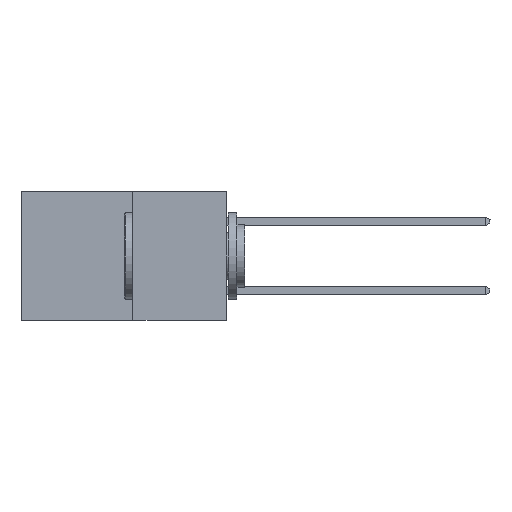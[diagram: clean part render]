
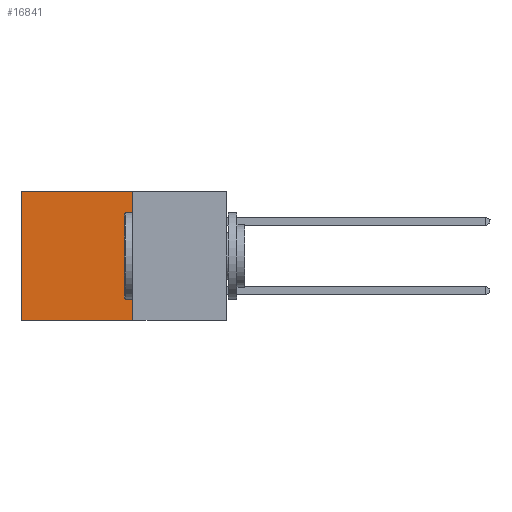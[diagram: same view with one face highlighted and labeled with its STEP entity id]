
A CAD part, left-side view. The second image highlights one B-rep face of the part: STEP entity #16841.
In plain terms, the highlighted planar face has unit normal (-1, 0, 0).
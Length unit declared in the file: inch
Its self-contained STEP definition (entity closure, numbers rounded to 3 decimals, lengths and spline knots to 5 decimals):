
#647 = VECTOR ( 'NONE', #2987, 39.37008 ) ;
#818 = DIRECTION ( 'NONE',  ( 0., 0., -1. ) ) ;
#966 = EDGE_CURVE ( 'NONE', #10498, #10838, #17862, .T. ) ;
#1390 = EDGE_LOOP ( 'NONE', ( #4282, #9911, #3294, #3325 ) ) ;
#2588 = CARTESIAN_POINT ( 'NONE',  ( 0.277, 0.27, -0.37 ) ) ;
#2857 = DIRECTION ( 'NONE',  ( 0., 1., 0. ) ) ;
#2987 = DIRECTION ( 'NONE',  ( 0., 0., -1. ) ) ;
#3294 = ORIENTED_EDGE ( 'NONE', *, *, #6069, .F. ) ;
#3325 = ORIENTED_EDGE ( 'NONE', *, *, #7299, .T. ) ;
#3700 = CARTESIAN_POINT ( 'NONE',  ( 0.277, 0.59, -0.37 ) ) ;
#3793 = LINE ( 'NONE', #2588, #647 ) ;
#3909 = AXIS2_PLACEMENT_3D ( 'NONE', #8554, #8508, #8469 ) ;
#4216 = VERTEX_POINT ( 'NONE', #9509 ) ;
#4282 = ORIENTED_EDGE ( 'NONE', *, *, #8366, .T. ) ;
#6069 = EDGE_CURVE ( 'NONE', #4216, #10498, #3793, .T. ) ;
#6804 = VECTOR ( 'NONE', #818, 39.37008 ) ;
#7299 = EDGE_CURVE ( 'NONE', #4216, #11428, #10470, .T. ) ;
#8366 = EDGE_CURVE ( 'NONE', #11428, #10838, #10786, .T. ) ;
#8469 = DIRECTION ( 'NONE',  ( 0., 0., -1. ) ) ;
#8508 = DIRECTION ( 'NONE',  ( 1., 0., 0. ) ) ;
#8554 = CARTESIAN_POINT ( 'NONE',  ( 0.277, 0.27, -0.37 ) ) ;
#8637 = PLANE ( 'NONE',  #3909 ) ;
#9115 = CARTESIAN_POINT ( 'NONE',  ( 0.277, 0.27, -0.37 ) ) ;
#9272 = CARTESIAN_POINT ( 'NONE',  ( 0.277, 0.59, 0. ) ) ;
#9509 = CARTESIAN_POINT ( 'NONE',  ( 0.277, 0.27, 0. ) ) ;
#9911 = ORIENTED_EDGE ( 'NONE', *, *, #966, .F. ) ;
#10009 = VECTOR ( 'NONE', #2857, 39.37008 ) ;
#10470 = LINE ( 'NONE', #14468, #10009 ) ;
#10498 = VERTEX_POINT ( 'NONE', #12800 ) ;
#10786 = LINE ( 'NONE', #3700, #6804 ) ;
#10838 = VERTEX_POINT ( 'NONE', #18921 ) ;
#11428 = VERTEX_POINT ( 'NONE', #9272 ) ;
#11753 = FACE_OUTER_BOUND ( 'NONE', #1390, .T. ) ;
#12800 = CARTESIAN_POINT ( 'NONE',  ( 0.277, 0.27, -0.37 ) ) ;
#14468 = CARTESIAN_POINT ( 'NONE',  ( 0.277, 0.27, 0. ) ) ;
#14542 = VECTOR ( 'NONE', #17769, 39.37008 ) ;
#16841 = ADVANCED_FACE ( 'NONE', ( #11753 ), #8637, .F. ) ;
#17769 = DIRECTION ( 'NONE',  ( 0., 1., 0. ) ) ;
#17862 = LINE ( 'NONE', #9115, #14542 ) ;
#18921 = CARTESIAN_POINT ( 'NONE',  ( 0.277, 0.59, -0.37 ) ) ;
